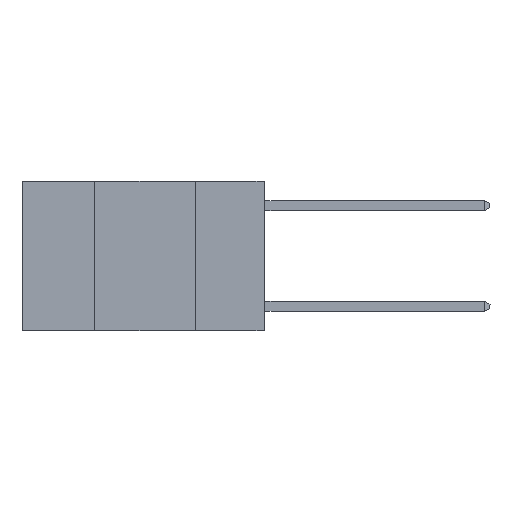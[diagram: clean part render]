
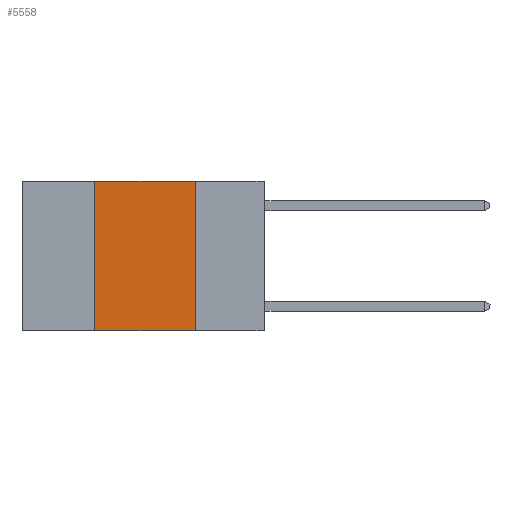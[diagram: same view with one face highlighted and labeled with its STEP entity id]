
A CAD part, left-side view. The second image highlights one B-rep face of the part: STEP entity #5558.
In plain terms, the highlighted planar face has unit normal (-1, 0, 0).
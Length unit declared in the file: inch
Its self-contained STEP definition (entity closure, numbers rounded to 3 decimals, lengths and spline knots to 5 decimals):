
#203 = CARTESIAN_POINT ( 'NONE',  ( 0., 0.6, -0.37 ) ) ;
#344 = EDGE_LOOP ( 'NONE', ( #5179, #9704, #6688, #4904 ) ) ;
#420 = CARTESIAN_POINT ( 'NONE',  ( 0., 0.42, -0.37 ) ) ;
#438 = CARTESIAN_POINT ( 'NONE',  ( 0., 0.17, 0. ) ) ;
#1195 = LINE ( 'NONE', #8918, #3763 ) ;
#1430 = CARTESIAN_POINT ( 'NONE',  ( 0., 0.17, 0. ) ) ;
#2262 = CARTESIAN_POINT ( 'NONE',  ( 0., 0.42, 0. ) ) ;
#2616 = LINE ( 'NONE', #203, #6408 ) ;
#2746 = VECTOR ( 'NONE', #5935, 39.37008 ) ;
#3514 = VERTEX_POINT ( 'NONE', #1430 ) ;
#3622 = EDGE_CURVE ( 'NONE', #6247, #6239, #2616, .T. ) ;
#3763 = VECTOR ( 'NONE', #3773, 39.37008 ) ;
#3773 = DIRECTION ( 'NONE',  ( 0., -1., 0. ) ) ;
#3844 = EDGE_CURVE ( 'NONE', #6247, #7031, #8658, .T. ) ;
#3874 = EDGE_CURVE ( 'NONE', #3514, #6239, #6301, .T. ) ;
#4228 = CARTESIAN_POINT ( 'NONE',  ( 0., 0.6, 0. ) ) ;
#4279 = VECTOR ( 'NONE', #4478, 39.37008 ) ;
#4478 = DIRECTION ( 'NONE',  ( 0., 0., -1. ) ) ;
#4904 = ORIENTED_EDGE ( 'NONE', *, *, #3622, .T. ) ;
#4941 = AXIS2_PLACEMENT_3D ( 'NONE', #4228, #9317, #5018 ) ;
#5018 = DIRECTION ( 'NONE',  ( 0., 0., -1. ) ) ;
#5179 = ORIENTED_EDGE ( 'NONE', *, *, #3874, .F. ) ;
#5558 = ADVANCED_FACE ( 'NONE', ( #7405 ), #8641, .F. ) ;
#5935 = DIRECTION ( 'NONE',  ( 0., 0., 1. ) ) ;
#6239 = VERTEX_POINT ( 'NONE', #6628 ) ;
#6247 = VERTEX_POINT ( 'NONE', #420 ) ;
#6301 = LINE ( 'NONE', #438, #4279 ) ;
#6408 = VECTOR ( 'NONE', #6441, 39.37008 ) ;
#6441 = DIRECTION ( 'NONE',  ( 0., -1., 0. ) ) ;
#6628 = CARTESIAN_POINT ( 'NONE',  ( 0., 0.17, -0.37 ) ) ;
#6688 = ORIENTED_EDGE ( 'NONE', *, *, #3844, .F. ) ;
#7031 = VERTEX_POINT ( 'NONE', #2262 ) ;
#7405 = FACE_OUTER_BOUND ( 'NONE', #344, .T. ) ;
#8641 = PLANE ( 'NONE',  #4941 ) ;
#8658 = LINE ( 'NONE', #9466, #2746 ) ;
#8918 = CARTESIAN_POINT ( 'NONE',  ( 0., 0.6, 0. ) ) ;
#8934 = EDGE_CURVE ( 'NONE', #7031, #3514, #1195, .T. ) ;
#9317 = DIRECTION ( 'NONE',  ( 1., 0., 0. ) ) ;
#9466 = CARTESIAN_POINT ( 'NONE',  ( 0., 0.42, 0. ) ) ;
#9704 = ORIENTED_EDGE ( 'NONE', *, *, #8934, .F. ) ;
